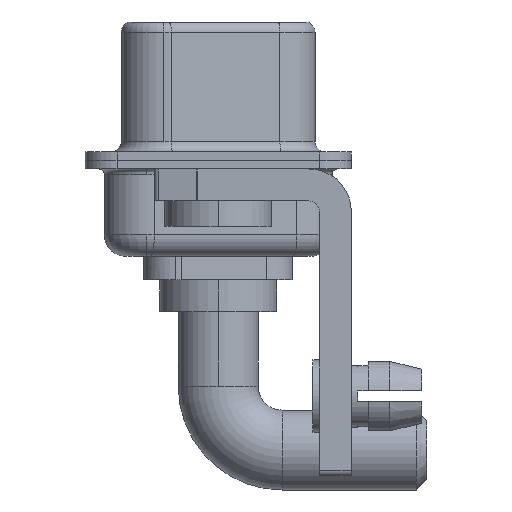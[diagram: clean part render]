
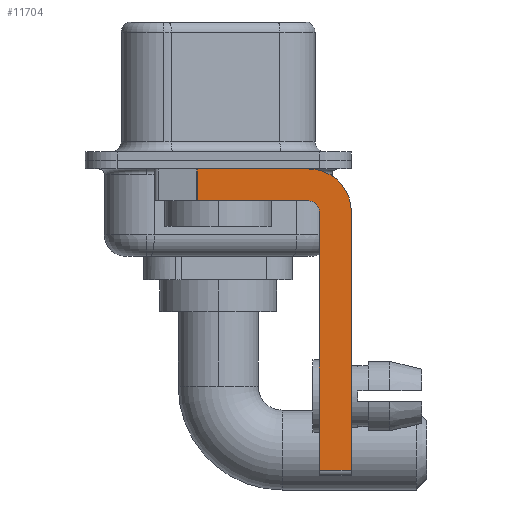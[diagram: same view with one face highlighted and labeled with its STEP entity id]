
A CAD part, left-side view. The second image highlights one B-rep face of the part: STEP entity #11704.
In plain terms, the highlighted planar face has unit normal (-1, 0, 0).
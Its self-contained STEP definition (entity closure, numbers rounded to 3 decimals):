
#658 = AXIS2_PLACEMENT_3D ( 'NONE', #15311, #9911, #15137 ) ;
#1204 = DIRECTION ( 'NONE',  ( 0., 0., -1. ) ) ;
#1385 = DIRECTION ( 'NONE',  ( 1., 0., 0. ) ) ;
#1484 = VERTEX_POINT ( 'NONE', #3033 ) ;
#1734 = DIRECTION ( 'NONE',  ( 1., 0., 0. ) ) ;
#1815 = CARTESIAN_POINT ( 'NONE',  ( -2.9, 0.978, -0.4 ) ) ;
#2095 = ORIENTED_EDGE ( 'NONE', *, *, #10091, .T. ) ;
#2122 = PLANE ( 'NONE',  #16112 ) ;
#2136 = VERTEX_POINT ( 'NONE', #6377 ) ;
#2169 = LINE ( 'NONE', #5036, #4512 ) ;
#3033 = CARTESIAN_POINT ( 'NONE',  ( -2.9, 0.978, -1.9 ) ) ;
#3330 = DIRECTION ( 'NONE',  ( 0., 0., -1. ) ) ;
#3581 = LINE ( 'NONE', #14305, #11005 ) ;
#3701 = VERTEX_POINT ( 'NONE', #8090 ) ;
#4271 = VECTOR ( 'NONE', #1204, 1000. ) ;
#4512 = VECTOR ( 'NONE', #12841, 1000. ) ;
#5036 = CARTESIAN_POINT ( 'NONE',  ( -2.9, -4.75, -14.8 ) ) ;
#5097 = CARTESIAN_POINT ( 'NONE',  ( -2.9, 0.978, -1.9 ) ) ;
#5601 = CARTESIAN_POINT ( 'NONE',  ( -2.9, -4.25, -0.4 ) ) ;
#5839 = VERTEX_POINT ( 'NONE', #5979 ) ;
#5896 = CIRCLE ( 'NONE', #658, 0.5 ) ;
#5979 = CARTESIAN_POINT ( 'NONE',  ( -2.9, -4.25, -1.9 ) ) ;
#6248 = ORIENTED_EDGE ( 'NONE', *, *, #14927, .F. ) ;
#6377 = CARTESIAN_POINT ( 'NONE',  ( -2.9, -6.25, -2.4 ) ) ;
#6583 = VERTEX_POINT ( 'NONE', #15075 ) ;
#6686 = VECTOR ( 'NONE', #11381, 1000. ) ;
#6821 = EDGE_CURVE ( 'NONE', #9726, #10271, #3581, .T. ) ;
#6922 = ORIENTED_EDGE ( 'NONE', *, *, #8860, .F. ) ;
#8090 = CARTESIAN_POINT ( 'NONE',  ( -2.9, -4.75, -2.4 ) ) ;
#8275 = CARTESIAN_POINT ( 'NONE',  ( -2.9, -4.25, -2.4 ) ) ;
#8288 = DIRECTION ( 'NONE',  ( 0., 0., -1. ) ) ;
#8673 = EDGE_LOOP ( 'NONE', ( #11946, #2095, #9858, #11104, #6248, #10975, #6922, #14059 ) ) ;
#8830 = DIRECTION ( 'NONE',  ( 0., -1., 0. ) ) ;
#8860 = EDGE_CURVE ( 'NONE', #2136, #10363, #14796, .T. ) ;
#9575 = EDGE_CURVE ( 'NONE', #10271, #2136, #10822, .T. ) ;
#9726 = VERTEX_POINT ( 'NONE', #1815 ) ;
#9809 = CARTESIAN_POINT ( 'NONE',  ( -2.9, -4.25, -14.55 ) ) ;
#9858 = ORIENTED_EDGE ( 'NONE', *, *, #10930, .F. ) ;
#9890 = EDGE_CURVE ( 'NONE', #6583, #10363, #15106, .T. ) ;
#9911 = DIRECTION ( 'NONE',  ( -1., 0., 0. ) ) ;
#9992 = VECTOR ( 'NONE', #15287, 1000. ) ;
#10091 = EDGE_CURVE ( 'NONE', #9726, #1484, #15704, .T. ) ;
#10182 = CARTESIAN_POINT ( 'NONE',  ( -2.9, -4.25, -1.9 ) ) ;
#10271 = VERTEX_POINT ( 'NONE', #5601 ) ;
#10363 = VERTEX_POINT ( 'NONE', #13895 ) ;
#10822 = CIRCLE ( 'NONE', #16555, 2. ) ;
#10930 = EDGE_CURVE ( 'NONE', #5839, #1484, #15327, .T. ) ;
#10975 = ORIENTED_EDGE ( 'NONE', *, *, #9890, .T. ) ;
#11005 = VECTOR ( 'NONE', #8830, 1000. ) ;
#11104 = ORIENTED_EDGE ( 'NONE', *, *, #15560, .F. ) ;
#11228 = FACE_OUTER_BOUND ( 'NONE', #8673, .T. ) ;
#11381 = DIRECTION ( 'NONE',  ( 0., 1., 0. ) ) ;
#11704 = ADVANCED_FACE ( 'NONE', ( #11228 ), #2122, .F. ) ;
#11946 = ORIENTED_EDGE ( 'NONE', *, *, #6821, .F. ) ;
#12588 = CARTESIAN_POINT ( 'NONE',  ( -2.9, -4.25, -2.4 ) ) ;
#12841 = DIRECTION ( 'NONE',  ( 0., 0., 1. ) ) ;
#13895 = CARTESIAN_POINT ( 'NONE',  ( -2.9, -6.25, -14.55 ) ) ;
#14059 = ORIENTED_EDGE ( 'NONE', *, *, #9575, .F. ) ;
#14305 = CARTESIAN_POINT ( 'NONE',  ( -2.9, 3., -0.4 ) ) ;
#14796 = LINE ( 'NONE', #15906, #15995 ) ;
#14927 = EDGE_CURVE ( 'NONE', #6583, #3701, #2169, .T. ) ;
#15075 = CARTESIAN_POINT ( 'NONE',  ( -2.9, -4.75, -14.55 ) ) ;
#15106 = LINE ( 'NONE', #9809, #9992 ) ;
#15137 = DIRECTION ( 'NONE',  ( 0., 0., 1. ) ) ;
#15287 = DIRECTION ( 'NONE',  ( 0., -1., 0. ) ) ;
#15311 = CARTESIAN_POINT ( 'NONE',  ( -2.9, -4.25, -2.4 ) ) ;
#15325 = DIRECTION ( 'NONE',  ( 0., 0., -1. ) ) ;
#15327 = LINE ( 'NONE', #10182, #6686 ) ;
#15560 = EDGE_CURVE ( 'NONE', #3701, #5839, #5896, .T. ) ;
#15704 = LINE ( 'NONE', #5097, #4271 ) ;
#15906 = CARTESIAN_POINT ( 'NONE',  ( -2.9, -6.25, -2.4 ) ) ;
#15995 = VECTOR ( 'NONE', #8288, 1000. ) ;
#16112 = AXIS2_PLACEMENT_3D ( 'NONE', #8275, #1734, #3330 ) ;
#16555 = AXIS2_PLACEMENT_3D ( 'NONE', #12588, #1385, #15325 ) ;
